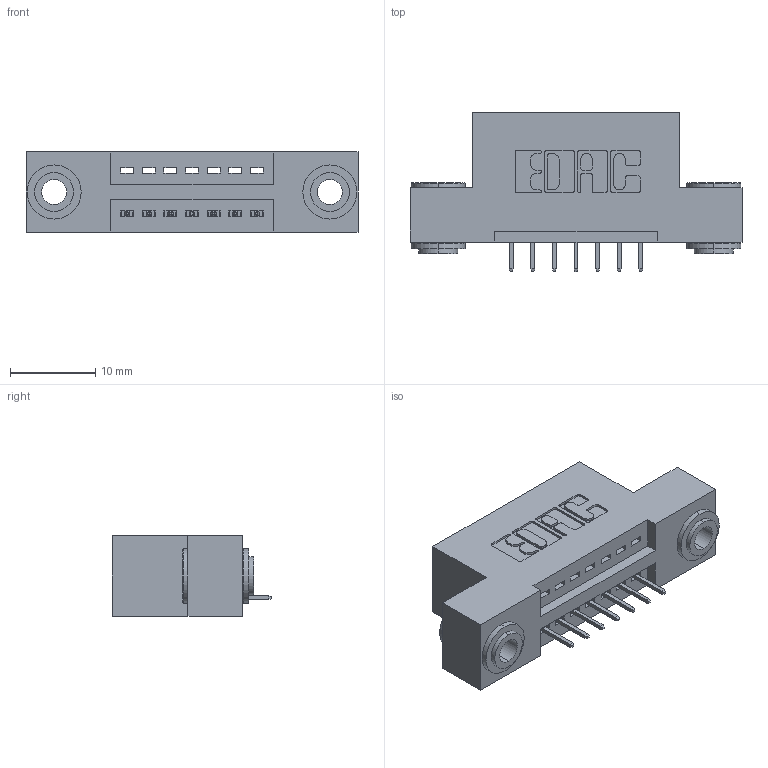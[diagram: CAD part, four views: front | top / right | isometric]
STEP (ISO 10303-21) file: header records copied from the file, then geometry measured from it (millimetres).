
FILE_DESCRIPTION (( 'STEP AP203' ), '1' );
FILE_NAME ('395-007-525-103.STEP', '2020-09-23T04:36:14', ( '' ), ( '' ), 'SwSTEP 2.0', 'SolidWorks 2020', '' );
FILE_SCHEMA (( 'CONFIG_CONTROL_DESIGN' ));
Length unit declared in the file: inch
Products named in the file (4): 395-007-525-103; 345 Part_Flush Mounting Lugs - 0.156 Dia-TH; 345-292-001_345-293-125; 345-250-002_345-250-002-102
Assembly tree (10 placements, depth 2):
  395-007-525-103
    345 Part_Flush Mounting Lugs - 0.156 Dia-TH
    345-292-001_345-293-125  x7
    345-250-002_345-250-002-102  x2
Bounding box: 38.99 x 18.72 x 9.4 mm (x, y, z)
Volume: 3407.3 mm3; surface area: 4171.5 mm2
Topology: 10 solids, 10 shells, 598 faces, 1677 edges, 1086 vertices
Faces by surface type: plane 412, cylinder 178, cone 8
Entity records: 10704 total; most frequent: CARTESIAN_POINT 1832, ORIENTED_EDGE 1766, DIRECTION 1683, EDGE_CURVE 883, VECTOR 703, LINE 703, VERTEX_POINT 582, AXIS2_PLACEMENT_3D 490
